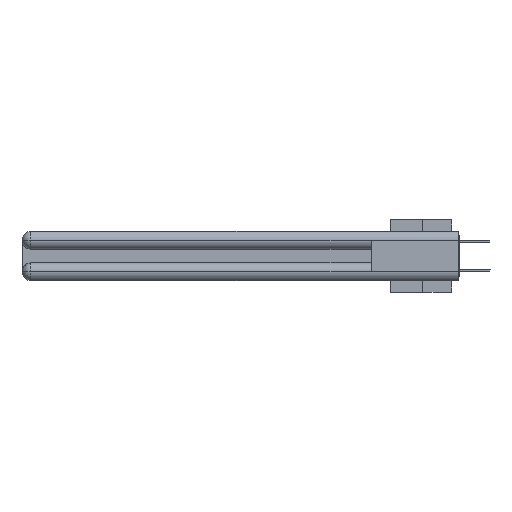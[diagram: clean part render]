
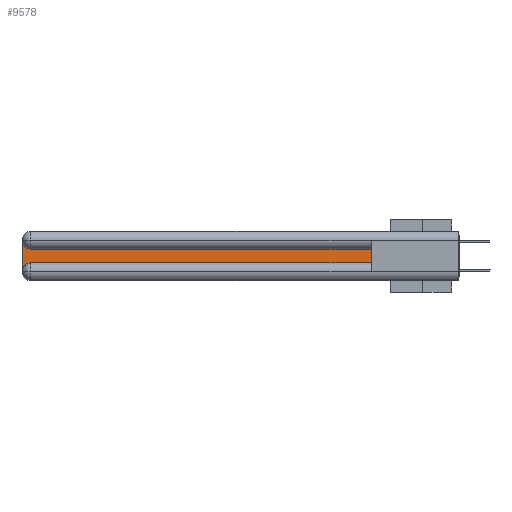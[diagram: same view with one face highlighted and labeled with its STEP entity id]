
A CAD part, left-side view. The second image highlights one B-rep face of the part: STEP entity #9578.
In plain terms, the highlighted planar face has unit normal (-1, 0, 0).
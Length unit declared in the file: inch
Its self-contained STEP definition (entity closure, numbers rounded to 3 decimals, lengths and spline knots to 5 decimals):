
#1603 = DIRECTION ( 'NONE',  ( 0., 0., -1. ) ) ;
#1925 = CARTESIAN_POINT ( 'NONE',  ( 0.075, 3., -0.0625 ) ) ;
#2559 = ORIENTED_EDGE ( 'NONE', *, *, #14015, .T. ) ;
#2826 = DIRECTION ( 'NONE',  ( 1., 0., 0. ) ) ;
#2909 = EDGE_CURVE ( 'NONE', #10449, #5162, #17738, .T. ) ;
#2964 = ORIENTED_EDGE ( 'NONE', *, *, #7505, .T. ) ;
#3995 = CARTESIAN_POINT ( 'NONE',  ( 0.075, 2.94, -0.0625 ) ) ;
#4091 = DIRECTION ( 'NONE',  ( 1., 0., 0. ) ) ;
#4473 = CARTESIAN_POINT ( 'NONE',  ( 0.075, 0.6, -0.1225 ) ) ;
#4557 = DIRECTION ( 'NONE',  ( 0., 0., 1. ) ) ;
#4558 = ORIENTED_EDGE ( 'NONE', *, *, #31075, .T. ) ;
#5162 = VERTEX_POINT ( 'NONE', #14671 ) ;
#5455 = VERTEX_POINT ( 'NONE', #1925 ) ;
#5792 = CARTESIAN_POINT ( 'NONE',  ( 0.075, 3., -0.1225 ) ) ;
#6403 = VERTEX_POINT ( 'NONE', #6824 ) ;
#6589 = VERTEX_POINT ( 'NONE', #21079 ) ;
#6824 = CARTESIAN_POINT ( 'NONE',  ( 0.075, 2.94, -0.1225 ) ) ;
#6840 = ORIENTED_EDGE ( 'NONE', *, *, #29494, .T. ) ;
#7505 = EDGE_CURVE ( 'NONE', #6589, #24060, #33611, .T. ) ;
#7732 = ORIENTED_EDGE ( 'NONE', *, *, #8720, .T. ) ;
#7739 = DIRECTION ( 'NONE',  ( 0., 0., -1. ) ) ;
#8220 = LINE ( 'NONE', #18615, #31055 ) ;
#8720 = EDGE_CURVE ( 'NONE', #5162, #6589, #8220, .T. ) ;
#9578 = ADVANCED_FACE ( 'NONE', ( #28057 ), #26359, .F. ) ;
#9975 = CARTESIAN_POINT ( 'NONE',  ( 0.075, 0.6, -0.2175 ) ) ;
#10449 = VERTEX_POINT ( 'NONE', #24430 ) ;
#10611 = CIRCLE ( 'NONE', #21787, 0.06 ) ;
#11579 = DIRECTION ( 'NONE',  ( 0., 0., -1. ) ) ;
#13386 = DIRECTION ( 'NONE',  ( 0., -1., 0. ) ) ;
#13519 = VECTOR ( 'NONE', #7739, 39.37008 ) ;
#14015 = EDGE_CURVE ( 'NONE', #5455, #10449, #28179, .T. ) ;
#14671 = CARTESIAN_POINT ( 'NONE',  ( 0.075, 2.94, -0.2175 ) ) ;
#17738 = CIRCLE ( 'NONE', #23689, 0.06 ) ;
#17920 = AXIS2_PLACEMENT_3D ( 'NONE', #5792, #32390, #24151 ) ;
#18615 = CARTESIAN_POINT ( 'NONE',  ( 0.075, 0.6, -0.2175 ) ) ;
#18698 = LINE ( 'NONE', #27045, #19899 ) ;
#19899 = VECTOR ( 'NONE', #21665, 39.37008 ) ;
#21079 = CARTESIAN_POINT ( 'NONE',  ( 0.075, 0.6, -0.2175 ) ) ;
#21665 = DIRECTION ( 'NONE',  ( 0., 1., 0. ) ) ;
#21787 = AXIS2_PLACEMENT_3D ( 'NONE', #3995, #4091, #11579 ) ;
#23689 = AXIS2_PLACEMENT_3D ( 'NONE', #31373, #2826, #1603 ) ;
#24060 = VERTEX_POINT ( 'NONE', #4473 ) ;
#24151 = DIRECTION ( 'NONE',  ( 0., 0., -1. ) ) ;
#24430 = CARTESIAN_POINT ( 'NONE',  ( 0.075, 3., -0.2775 ) ) ;
#24705 = EDGE_LOOP ( 'NONE', ( #4558, #6840, #2559, #33492, #7732, #2964 ) ) ;
#25765 = CARTESIAN_POINT ( 'NONE',  ( 0.075, 3., -0.2175 ) ) ;
#26359 = PLANE ( 'NONE',  #17920 ) ;
#27045 = CARTESIAN_POINT ( 'NONE',  ( 0.075, 0.6, -0.1225 ) ) ;
#28057 = FACE_OUTER_BOUND ( 'NONE', #24705, .T. ) ;
#28179 = LINE ( 'NONE', #25765, #13519 ) ;
#28289 = VECTOR ( 'NONE', #4557, 39.37008 ) ;
#29494 = EDGE_CURVE ( 'NONE', #6403, #5455, #10611, .T. ) ;
#31055 = VECTOR ( 'NONE', #13386, 39.37008 ) ;
#31075 = EDGE_CURVE ( 'NONE', #24060, #6403, #18698, .T. ) ;
#31373 = CARTESIAN_POINT ( 'NONE',  ( 0.075, 2.94, -0.2775 ) ) ;
#32390 = DIRECTION ( 'NONE',  ( 1., 0., 0. ) ) ;
#33492 = ORIENTED_EDGE ( 'NONE', *, *, #2909, .T. ) ;
#33611 = LINE ( 'NONE', #9975, #28289 ) ;
